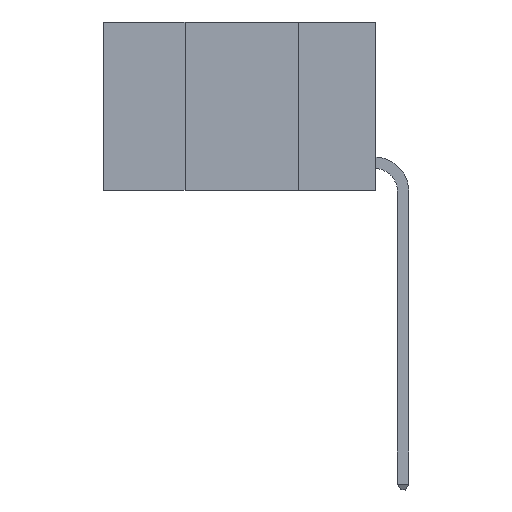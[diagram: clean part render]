
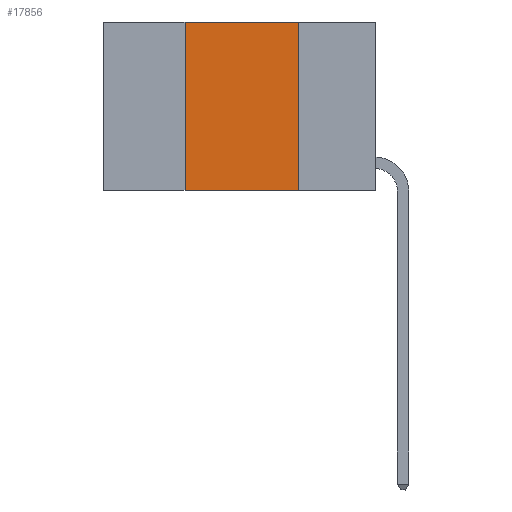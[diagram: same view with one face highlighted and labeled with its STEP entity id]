
A CAD part, left-side view. The second image highlights one B-rep face of the part: STEP entity #17856.
In plain terms, the highlighted planar face has unit normal (-1, 0, 0).
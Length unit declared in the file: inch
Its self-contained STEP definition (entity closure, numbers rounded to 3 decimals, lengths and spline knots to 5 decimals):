
#203 = PLANE ( 'NONE',  #18833 ) ;
#304 = CARTESIAN_POINT ( 'NONE',  ( 0., 0.6, -0.37 ) ) ;
#581 = LINE ( 'NONE', #15494, #14074 ) ;
#1671 = CARTESIAN_POINT ( 'NONE',  ( 0., 0.42, 0. ) ) ;
#1856 = CARTESIAN_POINT ( 'NONE',  ( 0., 0.17, 0. ) ) ;
#3498 = DIRECTION ( 'NONE',  ( 0., 0., 1. ) ) ;
#3767 = DIRECTION ( 'NONE',  ( 1., 0., 0. ) ) ;
#4115 = ORIENTED_EDGE ( 'NONE', *, *, #10044, .T. ) ;
#5217 = VECTOR ( 'NONE', #19678, 39.37008 ) ;
#5478 = VECTOR ( 'NONE', #3498, 39.37008 ) ;
#6301 = VECTOR ( 'NONE', #9122, 39.37008 ) ;
#7259 = EDGE_CURVE ( 'NONE', #16174, #21521, #581, .T. ) ;
#8134 = EDGE_CURVE ( 'NONE', #21521, #8358, #10495, .T. ) ;
#8358 = VERTEX_POINT ( 'NONE', #18581 ) ;
#8549 = DIRECTION ( 'NONE',  ( 0., -1., 0. ) ) ;
#9122 = DIRECTION ( 'NONE',  ( 0., -1., 0. ) ) ;
#9436 = CARTESIAN_POINT ( 'NONE',  ( 0., 0.17, 0. ) ) ;
#10044 = EDGE_CURVE ( 'NONE', #16083, #8358, #20033, .T. ) ;
#10159 = ORIENTED_EDGE ( 'NONE', *, *, #8134, .F. ) ;
#10495 = LINE ( 'NONE', #9436, #5217 ) ;
#11373 = ORIENTED_EDGE ( 'NONE', *, *, #7259, .F. ) ;
#11848 = LINE ( 'NONE', #1671, #5478 ) ;
#11933 = ORIENTED_EDGE ( 'NONE', *, *, #18363, .F. ) ;
#14074 = VECTOR ( 'NONE', #8549, 39.37008 ) ;
#15494 = CARTESIAN_POINT ( 'NONE',  ( 0., 0.6, 0. ) ) ;
#16048 = DIRECTION ( 'NONE',  ( 0., 0., -1. ) ) ;
#16083 = VERTEX_POINT ( 'NONE', #19837 ) ;
#16174 = VERTEX_POINT ( 'NONE', #20049 ) ;
#17491 = FACE_OUTER_BOUND ( 'NONE', #17817, .T. ) ;
#17817 = EDGE_LOOP ( 'NONE', ( #10159, #11373, #11933, #4115 ) ) ;
#17856 = ADVANCED_FACE ( 'NONE', ( #17491 ), #203, .F. ) ;
#18363 = EDGE_CURVE ( 'NONE', #16083, #16174, #11848, .T. ) ;
#18581 = CARTESIAN_POINT ( 'NONE',  ( 0., 0.17, -0.37 ) ) ;
#18833 = AXIS2_PLACEMENT_3D ( 'NONE', #19287, #3767, #16048 ) ;
#19287 = CARTESIAN_POINT ( 'NONE',  ( 0., 0.6, 0. ) ) ;
#19678 = DIRECTION ( 'NONE',  ( 0., 0., -1. ) ) ;
#19837 = CARTESIAN_POINT ( 'NONE',  ( 0., 0.42, -0.37 ) ) ;
#20033 = LINE ( 'NONE', #304, #6301 ) ;
#20049 = CARTESIAN_POINT ( 'NONE',  ( 0., 0.42, 0. ) ) ;
#21521 = VERTEX_POINT ( 'NONE', #1856 ) ;
